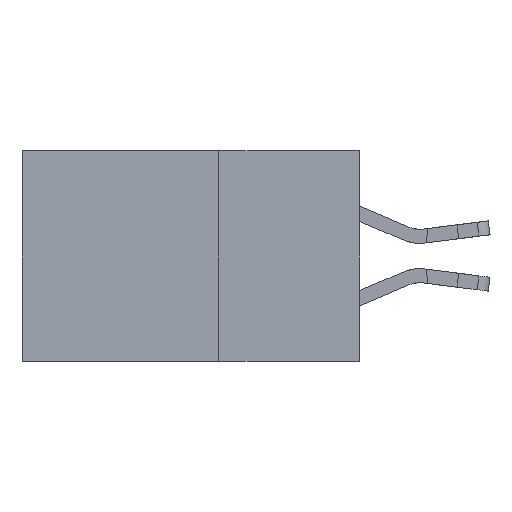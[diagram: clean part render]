
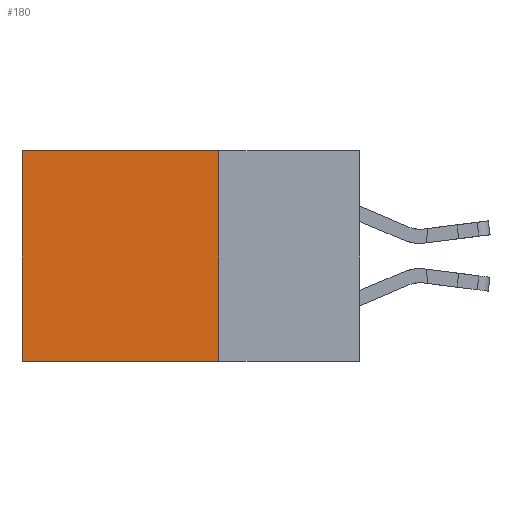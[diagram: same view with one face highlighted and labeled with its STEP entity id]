
A CAD part, left-side view. The second image highlights one B-rep face of the part: STEP entity #180.
In plain terms, the highlighted planar face has unit normal (-1, 0, 0).
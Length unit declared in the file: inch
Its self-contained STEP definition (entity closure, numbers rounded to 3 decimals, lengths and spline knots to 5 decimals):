
#116 = LINE ( 'NONE', #9805, #660 ) ;
#180 = ADVANCED_FACE ( 'NONE', ( #9101 ), #13576, .F. ) ;
#340 = DIRECTION ( 'NONE',  ( 1., 0., 0. ) ) ;
#660 = VECTOR ( 'NONE', #4442, 39.37008 ) ;
#715 = CARTESIAN_POINT ( 'NONE',  ( 0.2875, 0.6, -0.375 ) ) ;
#853 = LINE ( 'NONE', #11831, #1868 ) ;
#1425 = VECTOR ( 'NONE', #6089, 39.37008 ) ;
#1721 = ORIENTED_EDGE ( 'NONE', *, *, #3315, .F. ) ;
#1770 = VERTEX_POINT ( 'NONE', #7937 ) ;
#1868 = VECTOR ( 'NONE', #7286, 39.37008 ) ;
#2395 = ORIENTED_EDGE ( 'NONE', *, *, #13875, .T. ) ;
#2727 = DIRECTION ( 'NONE',  ( 0., 0., -1. ) ) ;
#3315 = EDGE_CURVE ( 'NONE', #1770, #6177, #853, .T. ) ;
#4012 = EDGE_LOOP ( 'NONE', ( #2395, #5966, #1721, #7431 ) ) ;
#4442 = DIRECTION ( 'NONE',  ( 0., 1., 0. ) ) ;
#5966 = ORIENTED_EDGE ( 'NONE', *, *, #6078, .F. ) ;
#6078 = EDGE_CURVE ( 'NONE', #6177, #11205, #9900, .T. ) ;
#6089 = DIRECTION ( 'NONE',  ( 0., 0., -1. ) ) ;
#6177 = VERTEX_POINT ( 'NONE', #7060 ) ;
#6229 = LINE ( 'NONE', #715, #1425 ) ;
#7049 = VERTEX_POINT ( 'NONE', #9153 ) ;
#7060 = CARTESIAN_POINT ( 'NONE',  ( 0.2875, 0.25, -0.375 ) ) ;
#7286 = DIRECTION ( 'NONE',  ( 0., 0., -1. ) ) ;
#7431 = ORIENTED_EDGE ( 'NONE', *, *, #8010, .T. ) ;
#7934 = VECTOR ( 'NONE', #7996, 39.37008 ) ;
#7937 = CARTESIAN_POINT ( 'NONE',  ( 0.2875, 0.25, 0. ) ) ;
#7996 = DIRECTION ( 'NONE',  ( 0., 1., 0. ) ) ;
#8010 = EDGE_CURVE ( 'NONE', #1770, #7049, #116, .T. ) ;
#8909 = CARTESIAN_POINT ( 'NONE',  ( 0.2875, 0.25, -0.375 ) ) ;
#9101 = FACE_OUTER_BOUND ( 'NONE', #4012, .T. ) ;
#9153 = CARTESIAN_POINT ( 'NONE',  ( 0.2875, 0.6, 0. ) ) ;
#9761 = CARTESIAN_POINT ( 'NONE',  ( 0.2875, 0.6, -0.375 ) ) ;
#9805 = CARTESIAN_POINT ( 'NONE',  ( 0.2875, 0.25, 0. ) ) ;
#9900 = LINE ( 'NONE', #8909, #7934 ) ;
#11205 = VERTEX_POINT ( 'NONE', #9761 ) ;
#11298 = CARTESIAN_POINT ( 'NONE',  ( 0.2875, 0.25, -0.375 ) ) ;
#11831 = CARTESIAN_POINT ( 'NONE',  ( 0.2875, 0.25, -0.375 ) ) ;
#13238 = AXIS2_PLACEMENT_3D ( 'NONE', #11298, #340, #2727 ) ;
#13576 = PLANE ( 'NONE',  #13238 ) ;
#13875 = EDGE_CURVE ( 'NONE', #7049, #11205, #6229, .T. ) ;
